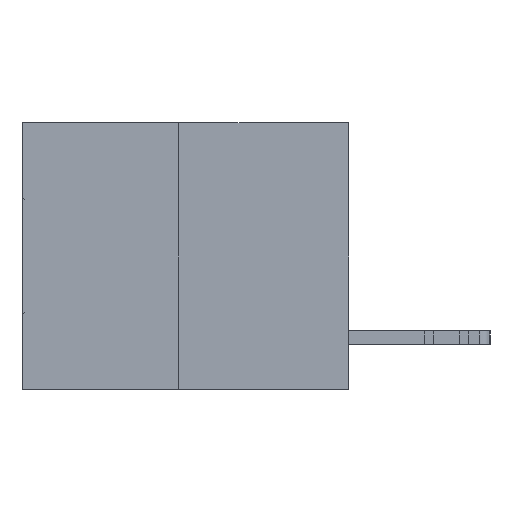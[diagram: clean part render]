
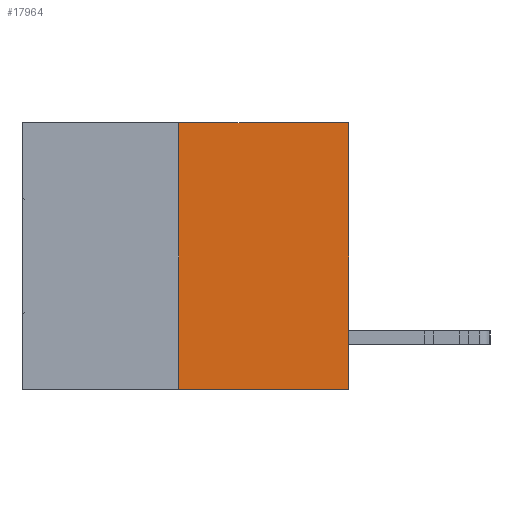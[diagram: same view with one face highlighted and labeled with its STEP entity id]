
A CAD part, left-side view. The second image highlights one B-rep face of the part: STEP entity #17964.
In plain terms, the highlighted planar face has unit normal (-1, 0, 0).
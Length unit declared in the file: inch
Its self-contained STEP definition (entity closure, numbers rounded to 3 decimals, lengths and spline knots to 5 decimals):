
#835 = VERTEX_POINT ( 'NONE', #24677 ) ;
#1597 = EDGE_CURVE ( 'NONE', #9611, #26613, #12914, .T. ) ;
#1714 = EDGE_CURVE ( 'NONE', #835, #26613, #22392, .T. ) ;
#2105 = AXIS2_PLACEMENT_3D ( 'NONE', #19905, #7390, #32578 ) ;
#4382 = CARTESIAN_POINT ( 'NONE',  ( 0., 0., -0.49 ) ) ;
#4659 = VECTOR ( 'NONE', #27123, 39.37008 ) ;
#5821 = ORIENTED_EDGE ( 'NONE', *, *, #1597, .T. ) ;
#6656 = CARTESIAN_POINT ( 'NONE',  ( 0., 0.312, -0.49 ) ) ;
#7390 = DIRECTION ( 'NONE',  ( 1., 0., 0. ) ) ;
#7488 = DIRECTION ( 'NONE',  ( 0., -1., 0. ) ) ;
#9611 = VERTEX_POINT ( 'NONE', #4382 ) ;
#11132 = DIRECTION ( 'NONE',  ( 0., 0., 1. ) ) ;
#12051 = ORIENTED_EDGE ( 'NONE', *, *, #1714, .F. ) ;
#12914 = LINE ( 'NONE', #22098, #4659 ) ;
#14045 = EDGE_CURVE ( 'NONE', #16695, #9611, #32477, .T. ) ;
#14883 = VECTOR ( 'NONE', #7488, 39.37008 ) ;
#14930 = DIRECTION ( 'NONE',  ( 0., -1., 0. ) ) ;
#15037 = CARTESIAN_POINT ( 'NONE',  ( 0., 0.6, -0.49 ) ) ;
#16015 = CARTESIAN_POINT ( 'NONE',  ( 0., 0., 0. ) ) ;
#16580 = EDGE_LOOP ( 'NONE', ( #31139, #24601, #5821, #12051 ) ) ;
#16695 = VERTEX_POINT ( 'NONE', #6656 ) ;
#17964 = ADVANCED_FACE ( 'NONE', ( #28721 ), #20006, .F. ) ;
#18916 = CARTESIAN_POINT ( 'NONE',  ( 0., 0.312, -0.49 ) ) ;
#19905 = CARTESIAN_POINT ( 'NONE',  ( 0., 0.6, 0. ) ) ;
#20006 = PLANE ( 'NONE',  #2105 ) ;
#20488 = LINE ( 'NONE', #18916, #32190 ) ;
#22098 = CARTESIAN_POINT ( 'NONE',  ( 0., 0., 0. ) ) ;
#22315 = VECTOR ( 'NONE', #14930, 39.37008 ) ;
#22392 = LINE ( 'NONE', #24956, #14883 ) ;
#24601 = ORIENTED_EDGE ( 'NONE', *, *, #14045, .T. ) ;
#24677 = CARTESIAN_POINT ( 'NONE',  ( 0., 0.312, 0. ) ) ;
#24956 = CARTESIAN_POINT ( 'NONE',  ( 0., 0.6, 0. ) ) ;
#26613 = VERTEX_POINT ( 'NONE', #16015 ) ;
#27123 = DIRECTION ( 'NONE',  ( 0., 0., 1. ) ) ;
#27288 = EDGE_CURVE ( 'NONE', #16695, #835, #20488, .T. ) ;
#28721 = FACE_OUTER_BOUND ( 'NONE', #16580, .T. ) ;
#31139 = ORIENTED_EDGE ( 'NONE', *, *, #27288, .F. ) ;
#32190 = VECTOR ( 'NONE', #11132, 39.37008 ) ;
#32477 = LINE ( 'NONE', #15037, #22315 ) ;
#32578 = DIRECTION ( 'NONE',  ( 0., 0., -1. ) ) ;
